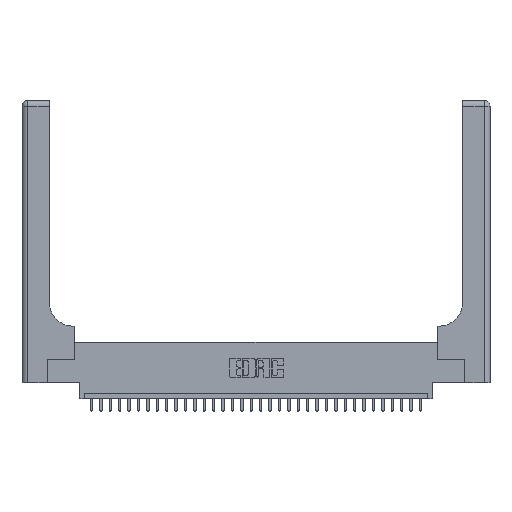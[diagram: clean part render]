
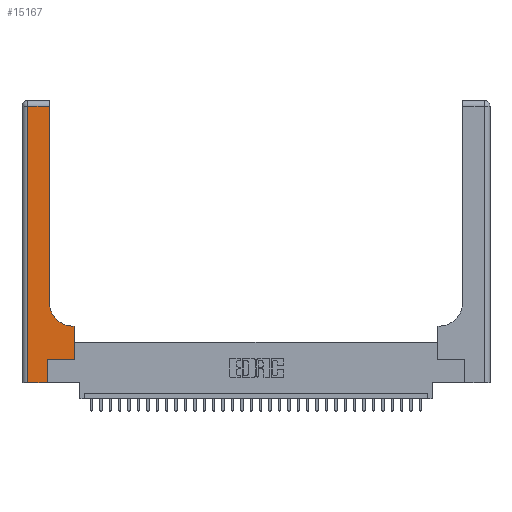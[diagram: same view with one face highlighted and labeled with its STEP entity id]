
A CAD part, top view. The second image highlights one B-rep face of the part: STEP entity #15167.
In plain terms, the highlighted planar face has unit normal (0, 0, 1).
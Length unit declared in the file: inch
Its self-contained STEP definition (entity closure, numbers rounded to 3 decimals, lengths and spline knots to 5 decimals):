
#349 = EDGE_CURVE ( 'NONE', #14703, #11234, #22489, .T. ) ;
#848 = AXIS2_PLACEMENT_3D ( 'NONE', #32329, #19562, #19675 ) ;
#933 = CARTESIAN_POINT ( 'NONE',  ( 0.269, 0., 0.37 ) ) ;
#1210 = VECTOR ( 'NONE', #23821, 39.37008 ) ;
#1514 = CARTESIAN_POINT ( 'NONE',  ( 0.2915, 3., 0.37 ) ) ;
#1862 = DIRECTION ( 'NONE',  ( -1., 0., 0. ) ) ;
#3283 = CIRCLE ( 'NONE', #848, 0.25 ) ;
#3574 = LINE ( 'NONE', #933, #33257 ) ;
#3600 = ORIENTED_EDGE ( 'NONE', *, *, #9467, .T. ) ;
#3641 = CARTESIAN_POINT ( 'NONE',  ( 0.06, 2.94, 0.37 ) ) ;
#3671 = VECTOR ( 'NONE', #14775, 39.37008 ) ;
#3846 = VERTEX_POINT ( 'NONE', #16413 ) ;
#3960 = DIRECTION ( 'NONE',  ( 0., -1., 0. ) ) ;
#5347 = CARTESIAN_POINT ( 'NONE',  ( 0.269, 0.25, 0.37 ) ) ;
#5668 = CARTESIAN_POINT ( 'NONE',  ( 0.06, 3., 0.37 ) ) ;
#6708 = CARTESIAN_POINT ( 'NONE',  ( 0., 3., 0.37 ) ) ;
#6934 = CARTESIAN_POINT ( 'NONE',  ( 0., 2.94, 0.37 ) ) ;
#7010 = DIRECTION ( 'NONE',  ( 0., 1., 0. ) ) ;
#7625 = EDGE_CURVE ( 'NONE', #13363, #32226, #11432, .T. ) ;
#7661 = CARTESIAN_POINT ( 'NONE',  ( 0.269, 0., 0.37 ) ) ;
#7850 = VECTOR ( 'NONE', #1862, 39.37008 ) ;
#7919 = CARTESIAN_POINT ( 'NONE',  ( 0.2915, 0.85, 0.37 ) ) ;
#8270 = CARTESIAN_POINT ( 'NONE',  ( 0.06, 0., 0.37 ) ) ;
#8656 = LINE ( 'NONE', #6934, #7850 ) ;
#9413 = EDGE_CURVE ( 'NONE', #11234, #30306, #3283, .T. ) ;
#9467 = EDGE_CURVE ( 'NONE', #32817, #23321, #24117, .T. ) ;
#9523 = EDGE_CURVE ( 'NONE', #14929, #13363, #23708, .T. ) ;
#9783 = ORIENTED_EDGE ( 'NONE', *, *, #9413, .T. ) ;
#11234 = VERTEX_POINT ( 'NONE', #21926 ) ;
#11245 = EDGE_CURVE ( 'NONE', #30306, #3846, #30870, .T. ) ;
#11432 = LINE ( 'NONE', #15486, #27445 ) ;
#13363 = VERTEX_POINT ( 'NONE', #8270 ) ;
#13932 = DIRECTION ( 'NONE',  ( 0., 1., 0. ) ) ;
#14401 = DIRECTION ( 'NONE',  ( 0., 0., -1. ) ) ;
#14479 = EDGE_LOOP ( 'NONE', ( #32134, #30653, #24645, #14585, #30093, #3600, #17504, #27235, #9783 ) ) ;
#14538 = CARTESIAN_POINT ( 'NONE',  ( 0.269, 0.25, 0.37 ) ) ;
#14585 = ORIENTED_EDGE ( 'NONE', *, *, #7625, .T. ) ;
#14703 = VERTEX_POINT ( 'NONE', #17812 ) ;
#14775 = DIRECTION ( 'NONE',  ( 1., 0., 0. ) ) ;
#14929 = VERTEX_POINT ( 'NONE', #3641 ) ;
#15167 = ADVANCED_FACE ( 'NONE', ( #30640 ), #22060, .F. ) ;
#15486 = CARTESIAN_POINT ( 'NONE',  ( 0., 0., 0.37 ) ) ;
#16413 = CARTESIAN_POINT ( 'NONE',  ( 0.2915, 2.94, 0.37 ) ) ;
#16864 = CARTESIAN_POINT ( 'NONE',  ( 0.5585, 0.25, 0.37 ) ) ;
#17244 = VECTOR ( 'NONE', #7010, 39.37008 ) ;
#17313 = DIRECTION ( 'NONE',  ( 1., 0., 0. ) ) ;
#17504 = ORIENTED_EDGE ( 'NONE', *, *, #31929, .T. ) ;
#17761 = CARTESIAN_POINT ( 'NONE',  ( 0.5585, 0.25, 0.37 ) ) ;
#17812 = CARTESIAN_POINT ( 'NONE',  ( 0.5585, 0.6, 0.37 ) ) ;
#18159 = AXIS2_PLACEMENT_3D ( 'NONE', #6708, #14401, #29876 ) ;
#19562 = DIRECTION ( 'NONE',  ( 0., 0., -1. ) ) ;
#19675 = DIRECTION ( 'NONE',  ( 1., 0., 0. ) ) ;
#19680 = DIRECTION ( 'NONE',  ( 0., 1., 0. ) ) ;
#20530 = VECTOR ( 'NONE', #3960, 39.37008 ) ;
#21926 = CARTESIAN_POINT ( 'NONE',  ( 0.5415, 0.6, 0.37 ) ) ;
#22060 = PLANE ( 'NONE',  #18159 ) ;
#22489 = LINE ( 'NONE', #27890, #1210 ) ;
#23231 = EDGE_CURVE ( 'NONE', #32226, #32817, #3574, .T. ) ;
#23321 = VERTEX_POINT ( 'NONE', #17761 ) ;
#23708 = LINE ( 'NONE', #5668, #20530 ) ;
#23821 = DIRECTION ( 'NONE',  ( -1., 0., 0. ) ) ;
#24117 = LINE ( 'NONE', #14538, #3671 ) ;
#24645 = ORIENTED_EDGE ( 'NONE', *, *, #9523, .T. ) ;
#25841 = LINE ( 'NONE', #16864, #26645 ) ;
#26645 = VECTOR ( 'NONE', #13932, 39.37008 ) ;
#27235 = ORIENTED_EDGE ( 'NONE', *, *, #349, .T. ) ;
#27445 = VECTOR ( 'NONE', #17313, 39.37008 ) ;
#27890 = CARTESIAN_POINT ( 'NONE',  ( 0.2915, 0.6, 0.37 ) ) ;
#29876 = DIRECTION ( 'NONE',  ( -1., 0., 0. ) ) ;
#30093 = ORIENTED_EDGE ( 'NONE', *, *, #23231, .T. ) ;
#30306 = VERTEX_POINT ( 'NONE', #7919 ) ;
#30640 = FACE_OUTER_BOUND ( 'NONE', #14479, .T. ) ;
#30653 = ORIENTED_EDGE ( 'NONE', *, *, #31381, .T. ) ;
#30870 = LINE ( 'NONE', #1514, #17244 ) ;
#31381 = EDGE_CURVE ( 'NONE', #3846, #14929, #8656, .T. ) ;
#31929 = EDGE_CURVE ( 'NONE', #23321, #14703, #25841, .T. ) ;
#32134 = ORIENTED_EDGE ( 'NONE', *, *, #11245, .T. ) ;
#32226 = VERTEX_POINT ( 'NONE', #7661 ) ;
#32329 = CARTESIAN_POINT ( 'NONE',  ( 0.5415, 0.85, 0.37 ) ) ;
#32817 = VERTEX_POINT ( 'NONE', #5347 ) ;
#33257 = VECTOR ( 'NONE', #19680, 39.37008 ) ;
